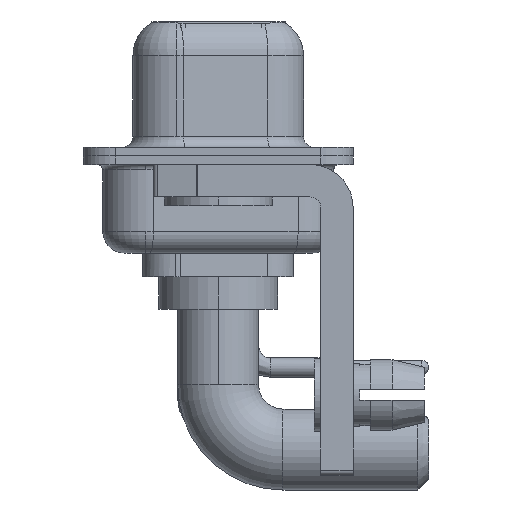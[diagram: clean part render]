
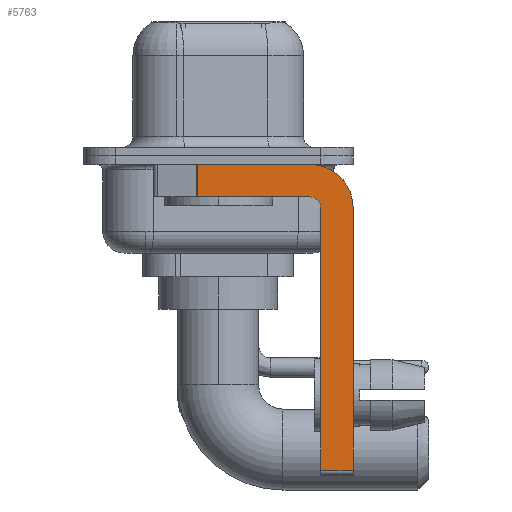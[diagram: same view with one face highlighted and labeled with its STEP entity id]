
A CAD part, left-side view. The second image highlights one B-rep face of the part: STEP entity #5763.
In plain terms, the highlighted planar face has unit normal (-1, 0, 0).
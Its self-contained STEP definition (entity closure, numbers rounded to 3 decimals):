
#103 = DIRECTION ( 'NONE',  ( 0., 0., -1. ) ) ;
#340 = EDGE_LOOP ( 'NONE', ( #9638, #21789, #8063, #19042, #4994, #3250, #12758, #11194 ) ) ;
#815 = CARTESIAN_POINT ( 'NONE',  ( -2.9, -4.25, -14.55 ) ) ;
#1125 = DIRECTION ( 'NONE',  ( 0., 1., 0. ) ) ;
#1407 = FACE_OUTER_BOUND ( 'NONE', #340, .T. ) ;
#2839 = CARTESIAN_POINT ( 'NONE',  ( -2.9, -6.25, -2.4 ) ) ;
#2902 = VERTEX_POINT ( 'NONE', #5716 ) ;
#3250 = ORIENTED_EDGE ( 'NONE', *, *, #14603, .T. ) ;
#3417 = CARTESIAN_POINT ( 'NONE',  ( -2.9, -4.25, -2.4 ) ) ;
#3504 = DIRECTION ( 'NONE',  ( 0., 0., -1. ) ) ;
#4060 = VERTEX_POINT ( 'NONE', #2839 ) ;
#4064 = VERTEX_POINT ( 'NONE', #10360 ) ;
#4994 = ORIENTED_EDGE ( 'NONE', *, *, #9969, .F. ) ;
#5192 = VERTEX_POINT ( 'NONE', #8039 ) ;
#5234 = DIRECTION ( 'NONE',  ( -1., 0., 0. ) ) ;
#5262 = LINE ( 'NONE', #11049, #11102 ) ;
#5304 = EDGE_CURVE ( 'NONE', #6154, #2902, #5262, .T. ) ;
#5468 = AXIS2_PLACEMENT_3D ( 'NONE', #14740, #5234, #22640 ) ;
#5716 = CARTESIAN_POINT ( 'NONE',  ( -2.9, -4.25, -0.4 ) ) ;
#5763 = ADVANCED_FACE ( 'NONE', ( #1407 ), #14975, .F. ) ;
#6154 = VERTEX_POINT ( 'NONE', #8287 ) ;
#6185 = EDGE_CURVE ( 'NONE', #8949, #5192, #8404, .T. ) ;
#7666 = EDGE_CURVE ( 'NONE', #4060, #4064, #22827, .T. ) ;
#8039 = CARTESIAN_POINT ( 'NONE',  ( -2.9, 0.978, -1.9 ) ) ;
#8063 = ORIENTED_EDGE ( 'NONE', *, *, #6185, .F. ) ;
#8287 = CARTESIAN_POINT ( 'NONE',  ( -2.9, 0.978, -0.4 ) ) ;
#8295 = VECTOR ( 'NONE', #9797, 1000. ) ;
#8404 = LINE ( 'NONE', #21638, #19929 ) ;
#8424 = CARTESIAN_POINT ( 'NONE',  ( -2.9, -4.75, -2.4 ) ) ;
#8476 = EDGE_CURVE ( 'NONE', #19159, #8949, #20835, .T. ) ;
#8949 = VERTEX_POINT ( 'NONE', #20637 ) ;
#9323 = DIRECTION ( 'NONE',  ( 0., 0., -1. ) ) ;
#9571 = CIRCLE ( 'NONE', #14725, 2. ) ;
#9638 = ORIENTED_EDGE ( 'NONE', *, *, #5304, .F. ) ;
#9797 = DIRECTION ( 'NONE',  ( 0., 0., 1. ) ) ;
#9969 = EDGE_CURVE ( 'NONE', #12703, #19159, #22672, .T. ) ;
#10032 = EDGE_CURVE ( 'NONE', #6154, #5192, #15121, .T. ) ;
#10360 = CARTESIAN_POINT ( 'NONE',  ( -2.9, -6.25, -14.55 ) ) ;
#11049 = CARTESIAN_POINT ( 'NONE',  ( -2.9, 3., -0.4 ) ) ;
#11102 = VECTOR ( 'NONE', #24284, 1000. ) ;
#11194 = ORIENTED_EDGE ( 'NONE', *, *, #17065, .F. ) ;
#11559 = CARTESIAN_POINT ( 'NONE',  ( -2.9, -6.25, -2.4 ) ) ;
#12703 = VERTEX_POINT ( 'NONE', #17026 ) ;
#12758 = ORIENTED_EDGE ( 'NONE', *, *, #7666, .F. ) ;
#14603 = EDGE_CURVE ( 'NONE', #12703, #4064, #15496, .T. ) ;
#14725 = AXIS2_PLACEMENT_3D ( 'NONE', #3417, #16747, #18605 ) ;
#14740 = CARTESIAN_POINT ( 'NONE',  ( -2.9, -4.25, -2.4 ) ) ;
#14975 = PLANE ( 'NONE',  #16776 ) ;
#15121 = LINE ( 'NONE', #22439, #17767 ) ;
#15496 = LINE ( 'NONE', #815, #22608 ) ;
#16747 = DIRECTION ( 'NONE',  ( 1., 0., 0. ) ) ;
#16776 = AXIS2_PLACEMENT_3D ( 'NONE', #20431, #20555, #3504 ) ;
#17026 = CARTESIAN_POINT ( 'NONE',  ( -2.9, -4.75, -14.55 ) ) ;
#17065 = EDGE_CURVE ( 'NONE', #2902, #4060, #9571, .T. ) ;
#17767 = VECTOR ( 'NONE', #9323, 1000. ) ;
#18605 = DIRECTION ( 'NONE',  ( 0., 0., -1. ) ) ;
#19042 = ORIENTED_EDGE ( 'NONE', *, *, #8476, .F. ) ;
#19159 = VERTEX_POINT ( 'NONE', #8424 ) ;
#19929 = VECTOR ( 'NONE', #1125, 1000. ) ;
#20431 = CARTESIAN_POINT ( 'NONE',  ( -2.9, -4.25, -2.4 ) ) ;
#20555 = DIRECTION ( 'NONE',  ( 1., 0., 0. ) ) ;
#20637 = CARTESIAN_POINT ( 'NONE',  ( -2.9, -4.25, -1.9 ) ) ;
#20835 = CIRCLE ( 'NONE', #5468, 0.5 ) ;
#21198 = VECTOR ( 'NONE', #103, 1000. ) ;
#21638 = CARTESIAN_POINT ( 'NONE',  ( -2.9, -4.25, -1.9 ) ) ;
#21789 = ORIENTED_EDGE ( 'NONE', *, *, #10032, .T. ) ;
#22439 = CARTESIAN_POINT ( 'NONE',  ( -2.9, 0.978, -1.9 ) ) ;
#22557 = CARTESIAN_POINT ( 'NONE',  ( -2.9, -4.75, -14.8 ) ) ;
#22608 = VECTOR ( 'NONE', #23045, 1000. ) ;
#22640 = DIRECTION ( 'NONE',  ( 0., 0., 1. ) ) ;
#22672 = LINE ( 'NONE', #22557, #8295 ) ;
#22827 = LINE ( 'NONE', #11559, #21198 ) ;
#23045 = DIRECTION ( 'NONE',  ( 0., -1., 0. ) ) ;
#24284 = DIRECTION ( 'NONE',  ( 0., -1., 0. ) ) ;
